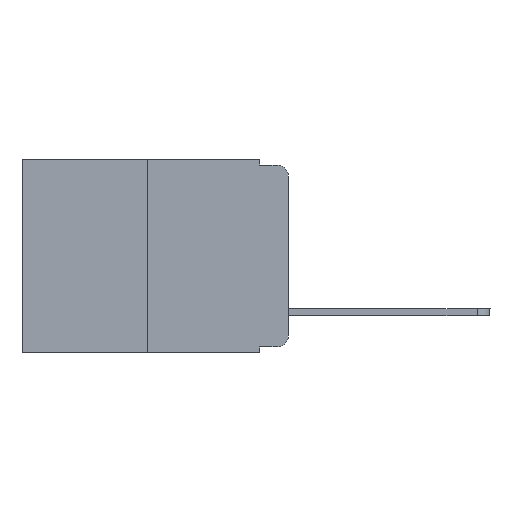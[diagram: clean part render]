
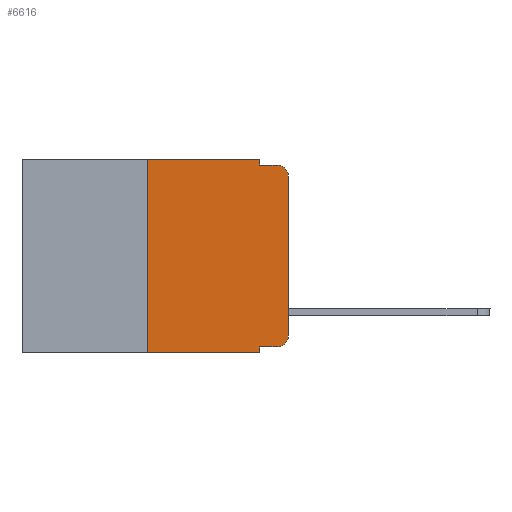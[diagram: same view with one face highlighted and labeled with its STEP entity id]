
A CAD part, left-side view. The second image highlights one B-rep face of the part: STEP entity #6616.
In plain terms, the highlighted planar face has unit normal (-1, 0, 0).
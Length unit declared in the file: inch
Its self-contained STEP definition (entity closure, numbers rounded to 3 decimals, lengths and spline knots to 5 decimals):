
#22 = VERTEX_POINT ( 'NONE', #2877 ) ;
#129 = DIRECTION ( 'NONE',  ( 0., 0., -1. ) ) ;
#346 = ORIENTED_EDGE ( 'NONE', *, *, #5850, .T. ) ;
#589 = ORIENTED_EDGE ( 'NONE', *, *, #5436, .F. ) ;
#607 = PLANE ( 'NONE',  #1186 ) ;
#653 = CARTESIAN_POINT ( 'NONE',  ( 0., 0.051, -0.333 ) ) ;
#981 = VECTOR ( 'NONE', #7001, 39.37008 ) ;
#1140 = LINE ( 'NONE', #4919, #4533 ) ;
#1186 = AXIS2_PLACEMENT_3D ( 'NONE', #9956, #3331, #10691 ) ;
#1204 = CIRCLE ( 'NONE', #3781, 0.02 ) ;
#1225 = DIRECTION ( 'NONE',  ( -1., 0., 0. ) ) ;
#1247 = VERTEX_POINT ( 'NONE', #5728 ) ;
#1513 = LINE ( 'NONE', #653, #8623 ) ;
#1586 = CARTESIAN_POINT ( 'NONE',  ( 0., 0.02, -0.333 ) ) ;
#1886 = DIRECTION ( 'NONE',  ( 0., -1., 0. ) ) ;
#2025 = VERTEX_POINT ( 'NONE', #7895 ) ;
#2147 = VECTOR ( 'NONE', #7283, 39.37008 ) ;
#2155 = VECTOR ( 'NONE', #6611, 39.37008 ) ;
#2276 = EDGE_CURVE ( 'NONE', #2895, #7138, #1513, .T. ) ;
#2877 = CARTESIAN_POINT ( 'NONE',  ( 0., 0.02, -0.01 ) ) ;
#2895 = VERTEX_POINT ( 'NONE', #9733 ) ;
#3331 = DIRECTION ( 'NONE',  ( 1., 0., 0. ) ) ;
#3489 = CARTESIAN_POINT ( 'NONE',  ( 0., 0.25, 0. ) ) ;
#3736 = CARTESIAN_POINT ( 'NONE',  ( 0., 0.051, -0.01 ) ) ;
#3781 = AXIS2_PLACEMENT_3D ( 'NONE', #4016, #1225, #129 ) ;
#3806 = DIRECTION ( 'NONE',  ( 0., 0., -1. ) ) ;
#4016 = CARTESIAN_POINT ( 'NONE',  ( 0., 0.02, -0.313 ) ) ;
#4100 = ORIENTED_EDGE ( 'NONE', *, *, #8946, .F. ) ;
#4278 = CARTESIAN_POINT ( 'NONE',  ( 0., 0.051, 0. ) ) ;
#4305 = VERTEX_POINT ( 'NONE', #4278 ) ;
#4424 = CARTESIAN_POINT ( 'NONE',  ( 0., 0., 0. ) ) ;
#4524 = CARTESIAN_POINT ( 'NONE',  ( 0., 0.02, -0.03 ) ) ;
#4533 = VECTOR ( 'NONE', #8704, 39.37008 ) ;
#4664 = CARTESIAN_POINT ( 'NONE',  ( 0., 0.051, 0. ) ) ;
#4719 = LINE ( 'NONE', #6602, #5555 ) ;
#4823 = ORIENTED_EDGE ( 'NONE', *, *, #2276, .T. ) ;
#4917 = VECTOR ( 'NONE', #8259, 39.37008 ) ;
#4919 = CARTESIAN_POINT ( 'NONE',  ( 0., 0.051, 0. ) ) ;
#4986 = ORIENTED_EDGE ( 'NONE', *, *, #5430, .F. ) ;
#5150 = EDGE_CURVE ( 'NONE', #1247, #9162, #11962, .T. ) ;
#5372 = LINE ( 'NONE', #4424, #4917 ) ;
#5381 = EDGE_CURVE ( 'NONE', #7445, #2025, #5372, .T. ) ;
#5430 = EDGE_CURVE ( 'NONE', #4305, #5991, #12147, .T. ) ;
#5436 = EDGE_CURVE ( 'NONE', #5991, #22, #11351, .T. ) ;
#5555 = VECTOR ( 'NONE', #1886, 39.37008 ) ;
#5728 = CARTESIAN_POINT ( 'NONE',  ( 0., 0.25, -0.343 ) ) ;
#5850 = EDGE_CURVE ( 'NONE', #2025, #22, #10055, .T. ) ;
#5991 = VERTEX_POINT ( 'NONE', #8613 ) ;
#6027 = EDGE_LOOP ( 'NONE', ( #9509, #346, #589, #4986, #4100, #6225, #8731, #9336, #4823, #12086 ) ) ;
#6189 = LINE ( 'NONE', #10673, #981 ) ;
#6225 = ORIENTED_EDGE ( 'NONE', *, *, #5150, .F. ) ;
#6602 = CARTESIAN_POINT ( 'NONE',  ( 0., 0.473, 0. ) ) ;
#6611 = DIRECTION ( 'NONE',  ( 0., -1., 0. ) ) ;
#6616 = ADVANCED_FACE ( 'NONE', ( #11803 ), #607, .F. ) ;
#6707 = VECTOR ( 'NONE', #3806, 39.37008 ) ;
#7001 = DIRECTION ( 'NONE',  ( 0., -1., 0. ) ) ;
#7025 = EDGE_CURVE ( 'NONE', #1247, #9499, #6189, .T. ) ;
#7109 = DIRECTION ( 'NONE',  ( 0., -1., 0. ) ) ;
#7138 = VERTEX_POINT ( 'NONE', #1586 ) ;
#7283 = DIRECTION ( 'NONE',  ( 0., 0., 1. ) ) ;
#7445 = VERTEX_POINT ( 'NONE', #8232 ) ;
#7520 = DIRECTION ( 'NONE',  ( 0., 0., -1. ) ) ;
#7895 = CARTESIAN_POINT ( 'NONE',  ( 0., 0., -0.03 ) ) ;
#8232 = CARTESIAN_POINT ( 'NONE',  ( 0., 0., -0.313 ) ) ;
#8259 = DIRECTION ( 'NONE',  ( 0., 0., 1. ) ) ;
#8537 = EDGE_CURVE ( 'NONE', #2895, #9499, #1140, .T. ) ;
#8613 = CARTESIAN_POINT ( 'NONE',  ( 0., 0.051, -0.01 ) ) ;
#8623 = VECTOR ( 'NONE', #7109, 39.37008 ) ;
#8704 = DIRECTION ( 'NONE',  ( 0., 0., -1. ) ) ;
#8731 = ORIENTED_EDGE ( 'NONE', *, *, #7025, .T. ) ;
#8946 = EDGE_CURVE ( 'NONE', #9162, #4305, #4719, .T. ) ;
#9162 = VERTEX_POINT ( 'NONE', #10558 ) ;
#9336 = ORIENTED_EDGE ( 'NONE', *, *, #8537, .F. ) ;
#9421 = DIRECTION ( 'NONE',  ( -1., 0., 0. ) ) ;
#9499 = VERTEX_POINT ( 'NONE', #10900 ) ;
#9509 = ORIENTED_EDGE ( 'NONE', *, *, #5381, .T. ) ;
#9733 = CARTESIAN_POINT ( 'NONE',  ( 0., 0.051, -0.333 ) ) ;
#9956 = CARTESIAN_POINT ( 'NONE',  ( 0., 0.473, 0. ) ) ;
#10055 = CIRCLE ( 'NONE', #10255, 0.02 ) ;
#10255 = AXIS2_PLACEMENT_3D ( 'NONE', #4524, #9421, #7520 ) ;
#10558 = CARTESIAN_POINT ( 'NONE',  ( 0., 0.25, 0. ) ) ;
#10673 = CARTESIAN_POINT ( 'NONE',  ( 0., 0.473, -0.343 ) ) ;
#10691 = DIRECTION ( 'NONE',  ( 0., 0., -1. ) ) ;
#10900 = CARTESIAN_POINT ( 'NONE',  ( 0., 0.051, -0.343 ) ) ;
#11351 = LINE ( 'NONE', #3736, #2155 ) ;
#11406 = EDGE_CURVE ( 'NONE', #7138, #7445, #1204, .T. ) ;
#11803 = FACE_OUTER_BOUND ( 'NONE', #6027, .T. ) ;
#11962 = LINE ( 'NONE', #3489, #2147 ) ;
#12086 = ORIENTED_EDGE ( 'NONE', *, *, #11406, .T. ) ;
#12147 = LINE ( 'NONE', #4664, #6707 ) ;
